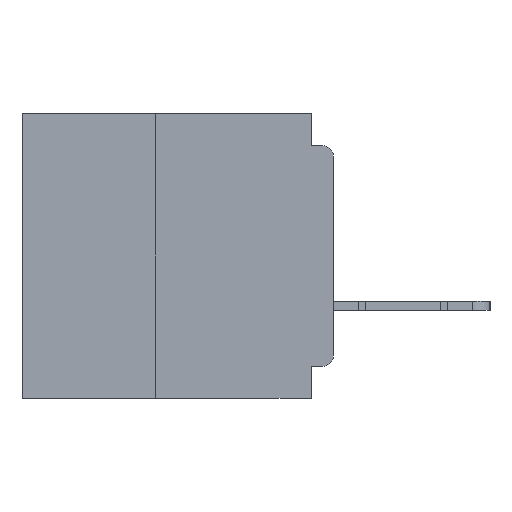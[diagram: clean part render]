
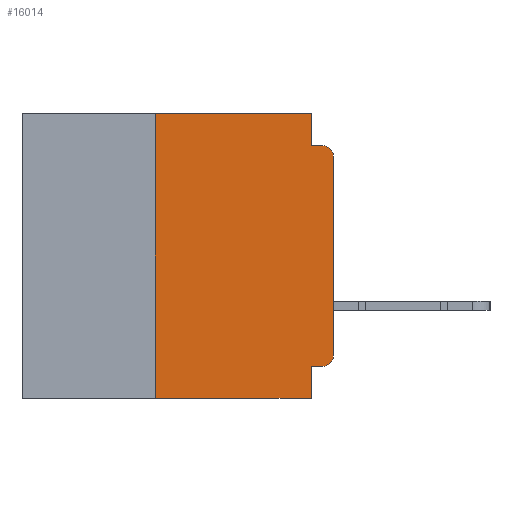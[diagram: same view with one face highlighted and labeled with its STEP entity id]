
A CAD part, left-side view. The second image highlights one B-rep face of the part: STEP entity #16014.
In plain terms, the highlighted planar face has unit normal (-1, 0, 0).
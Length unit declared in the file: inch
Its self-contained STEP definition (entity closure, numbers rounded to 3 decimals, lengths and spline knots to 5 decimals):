
#655 = DIRECTION ( 'NONE',  ( 0., 0., -1. ) ) ;
#1050 = DIRECTION ( 'NONE',  ( -1., 0., 0. ) ) ;
#1305 = CARTESIAN_POINT ( 'NONE',  ( 0., 0.031, -0.045 ) ) ;
#2290 = CARTESIAN_POINT ( 'NONE',  ( 0., 0.25, -0.4 ) ) ;
#5943 = VECTOR ( 'NONE', #63389, 39.37008 ) ;
#6244 = CARTESIAN_POINT ( 'NONE',  ( 0., 0.437, -0.4 ) ) ;
#7315 = EDGE_CURVE ( 'NONE', #13958, #61876, #14430, .T. ) ;
#9447 = DIRECTION ( 'NONE',  ( 1., 0., 0. ) ) ;
#9692 = EDGE_CURVE ( 'NONE', #15000, #61912, #33353, .T. ) ;
#10964 = VERTEX_POINT ( 'NONE', #54632 ) ;
#11671 = DIRECTION ( 'NONE',  ( 0., 1., 0. ) ) ;
#12410 = VECTOR ( 'NONE', #17302, 39.37008 ) ;
#12884 = CIRCLE ( 'NONE', #30704, 0.015 ) ;
#12941 = DIRECTION ( 'NONE',  ( 0., 0., 1. ) ) ;
#13958 = VERTEX_POINT ( 'NONE', #53299 ) ;
#14058 = CARTESIAN_POINT ( 'NONE',  ( 0., 0.437, 0. ) ) ;
#14430 = LINE ( 'NONE', #42277, #16064 ) ;
#14729 = EDGE_LOOP ( 'NONE', ( #38353, #25384, #48832, #37007, #49226, #42453, #22704, #32546, #33552, #46088 ) ) ;
#14746 = LINE ( 'NONE', #23124, #37146 ) ;
#15000 = VERTEX_POINT ( 'NONE', #1305 ) ;
#16014 = ADVANCED_FACE ( 'NONE', ( #32726 ), #65130, .F. ) ;
#16064 = VECTOR ( 'NONE', #11671, 39.37008 ) ;
#16899 = CARTESIAN_POINT ( 'NONE',  ( 0., 0.015, -0.34 ) ) ;
#17302 = DIRECTION ( 'NONE',  ( 0., 0., 1. ) ) ;
#18123 = CARTESIAN_POINT ( 'NONE',  ( 0., 0., -0.34 ) ) ;
#18214 = VECTOR ( 'NONE', #37021, 39.37008 ) ;
#20018 = EDGE_CURVE ( 'NONE', #61876, #10964, #63736, .T. ) ;
#22109 = DIRECTION ( 'NONE',  ( 0., 0., -1. ) ) ;
#22512 = CARTESIAN_POINT ( 'NONE',  ( 0., 0., 0. ) ) ;
#22704 = ORIENTED_EDGE ( 'NONE', *, *, #47846, .T. ) ;
#23124 = CARTESIAN_POINT ( 'NONE',  ( 0., 0.25, -0.4 ) ) ;
#25384 = ORIENTED_EDGE ( 'NONE', *, *, #52602, .T. ) ;
#27566 = EDGE_CURVE ( 'NONE', #13958, #60121, #42238, .T. ) ;
#27774 = CARTESIAN_POINT ( 'NONE',  ( 0., 0., -0.045 ) ) ;
#29350 = CARTESIAN_POINT ( 'NONE',  ( 0., 0.031, 0. ) ) ;
#30564 = AXIS2_PLACEMENT_3D ( 'NONE', #40101, #9447, #45140 ) ;
#30704 = AXIS2_PLACEMENT_3D ( 'NONE', #32018, #1050, #37109 ) ;
#31316 = VERTEX_POINT ( 'NONE', #2290 ) ;
#31641 = CARTESIAN_POINT ( 'NONE',  ( 0., 0.031, 0. ) ) ;
#31810 = LINE ( 'NONE', #6244, #18214 ) ;
#32018 = CARTESIAN_POINT ( 'NONE',  ( 0., 0.015, -0.06 ) ) ;
#32546 = ORIENTED_EDGE ( 'NONE', *, *, #20018, .F. ) ;
#32726 = FACE_OUTER_BOUND ( 'NONE', #14729, .T. ) ;
#33353 = LINE ( 'NONE', #27774, #5943 ) ;
#33552 = ORIENTED_EDGE ( 'NONE', *, *, #7315, .F. ) ;
#35781 = CARTESIAN_POINT ( 'NONE',  ( 0., 0.031, -0.4 ) ) ;
#36838 = VECTOR ( 'NONE', #66090, 39.37008 ) ;
#37007 = ORIENTED_EDGE ( 'NONE', *, *, #43566, .F. ) ;
#37021 = DIRECTION ( 'NONE',  ( 0., -1., 0. ) ) ;
#37109 = DIRECTION ( 'NONE',  ( 0., 0., -1. ) ) ;
#37146 = VECTOR ( 'NONE', #12941, 39.37008 ) ;
#37398 = VERTEX_POINT ( 'NONE', #29350 ) ;
#38353 = ORIENTED_EDGE ( 'NONE', *, *, #50289, .T. ) ;
#39850 = VERTEX_POINT ( 'NONE', #49590 ) ;
#40101 = CARTESIAN_POINT ( 'NONE',  ( 0., 0.437, 0. ) ) ;
#42238 = CIRCLE ( 'NONE', #49297, 0.015 ) ;
#42277 = CARTESIAN_POINT ( 'NONE',  ( 0., 0., -0.355 ) ) ;
#42453 = ORIENTED_EDGE ( 'NONE', *, *, #50876, .F. ) ;
#42772 = LINE ( 'NONE', #22512, #12410 ) ;
#43566 = EDGE_CURVE ( 'NONE', #37398, #15000, #49437, .T. ) ;
#45140 = DIRECTION ( 'NONE',  ( 0., 0., -1. ) ) ;
#46088 = ORIENTED_EDGE ( 'NONE', *, *, #27566, .T. ) ;
#46969 = EDGE_CURVE ( 'NONE', #60247, #37398, #48497, .T. ) ;
#47846 = EDGE_CURVE ( 'NONE', #31316, #10964, #31810, .T. ) ;
#48497 = LINE ( 'NONE', #14058, #62008 ) ;
#48832 = ORIENTED_EDGE ( 'NONE', *, *, #9692, .F. ) ;
#49226 = ORIENTED_EDGE ( 'NONE', *, *, #46969, .F. ) ;
#49297 = AXIS2_PLACEMENT_3D ( 'NONE', #16899, #52377, #22109 ) ;
#49437 = LINE ( 'NONE', #31641, #51014 ) ;
#49590 = CARTESIAN_POINT ( 'NONE',  ( 0., 0., -0.06 ) ) ;
#50289 = EDGE_CURVE ( 'NONE', #60121, #39850, #42772, .T. ) ;
#50876 = EDGE_CURVE ( 'NONE', #31316, #60247, #14746, .T. ) ;
#51014 = VECTOR ( 'NONE', #655, 39.37008 ) ;
#52377 = DIRECTION ( 'NONE',  ( -1., 0., 0. ) ) ;
#52602 = EDGE_CURVE ( 'NONE', #39850, #61912, #12884, .T. ) ;
#53299 = CARTESIAN_POINT ( 'NONE',  ( 0., 0.015, -0.355 ) ) ;
#54632 = CARTESIAN_POINT ( 'NONE',  ( 0., 0.031, -0.4 ) ) ;
#60121 = VERTEX_POINT ( 'NONE', #18123 ) ;
#60247 = VERTEX_POINT ( 'NONE', #64508 ) ;
#61876 = VERTEX_POINT ( 'NONE', #63355 ) ;
#61912 = VERTEX_POINT ( 'NONE', #63578 ) ;
#62008 = VECTOR ( 'NONE', #64773, 39.37008 ) ;
#63355 = CARTESIAN_POINT ( 'NONE',  ( 0., 0.031, -0.355 ) ) ;
#63389 = DIRECTION ( 'NONE',  ( 0., -1., 0. ) ) ;
#63578 = CARTESIAN_POINT ( 'NONE',  ( 0., 0.015, -0.045 ) ) ;
#63736 = LINE ( 'NONE', #35781, #36838 ) ;
#64508 = CARTESIAN_POINT ( 'NONE',  ( 0., 0.25, 0. ) ) ;
#64773 = DIRECTION ( 'NONE',  ( 0., -1., 0. ) ) ;
#65130 = PLANE ( 'NONE',  #30564 ) ;
#66090 = DIRECTION ( 'NONE',  ( 0., 0., -1. ) ) ;
